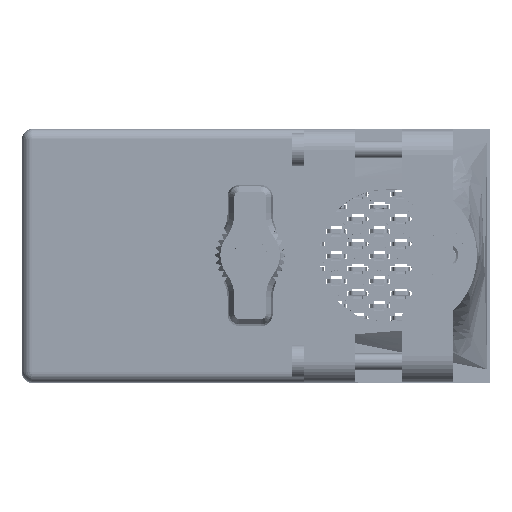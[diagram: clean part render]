
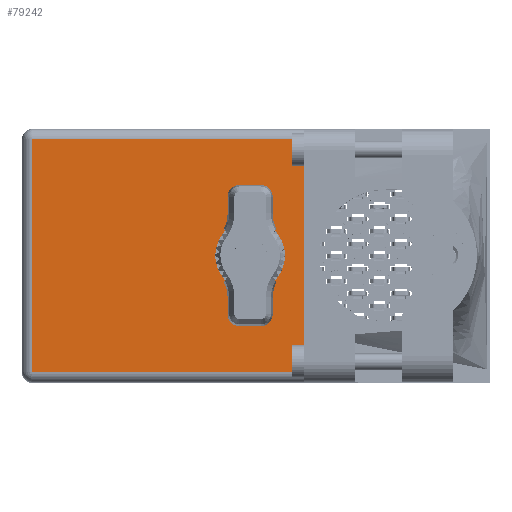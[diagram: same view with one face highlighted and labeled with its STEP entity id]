
A CAD part, top view. The second image highlights one B-rep face of the part: STEP entity #79242.
In plain terms, the highlighted face is planar.
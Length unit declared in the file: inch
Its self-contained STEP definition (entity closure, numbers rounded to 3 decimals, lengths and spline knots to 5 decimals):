
#1709 = DIRECTION ( 'NONE',  ( -1., 0., 0. ) ) ;
#2238 = EDGE_CURVE ( 'NONE', #68252, #86363, #70495, .T. ) ;
#2355 = VERTEX_POINT ( 'NONE', #63988 ) ;
#6141 = EDGE_CURVE ( 'NONE', #2355, #67868, #67649, .T. ) ;
#7275 = CARTESIAN_POINT ( 'NONE',  ( 0.3275, 1.93, 0.703 ) ) ;
#8438 = EDGE_CURVE ( 'NONE', #25638, #2355, #34838, .T. ) ;
#10972 = DIRECTION ( 'NONE',  ( 0., 0., 1. ) ) ;
#18966 = DIRECTION ( 'NONE',  ( 0., 0., 1. ) ) ;
#19156 = AXIS2_PLACEMENT_3D ( 'NONE', #27932, #29498, #1709 ) ;
#25561 = DIRECTION ( 'NONE',  ( 0., 0., 1. ) ) ;
#25638 = VERTEX_POINT ( 'NONE', #112360 ) ;
#27932 = CARTESIAN_POINT ( 'NONE',  ( -1.3775, 1.93, -0.765 ) ) ;
#28512 = EDGE_LOOP ( 'NONE', ( #109829, #52569, #81997, #28928 ) ) ;
#28665 = DIRECTION ( 'NONE',  ( 0., 0., 1. ) ) ;
#28928 = ORIENTED_EDGE ( 'NONE', *, *, #32150, .T. ) ;
#29498 = DIRECTION ( 'NONE',  ( 0., 1., 0. ) ) ;
#29762 = CARTESIAN_POINT ( 'NONE',  ( -1.3155, 1.93, -0.765 ) ) ;
#32150 = EDGE_CURVE ( 'NONE', #102477, #25638, #57107, .T. ) ;
#33489 = AXIS2_PLACEMENT_3D ( 'NONE', #60456, #79254, #25561 ) ;
#34838 = LINE ( 'NONE', #29762, #99309 ) ;
#41670 = CARTESIAN_POINT ( 'NONE',  ( 0.3275, 1.93, -0.703 ) ) ;
#45185 = FACE_OUTER_BOUND ( 'NONE', #28512, .T. ) ;
#47672 = CARTESIAN_POINT ( 'NONE',  ( -1.3775, 1.93, -0.703 ) ) ;
#47710 = CARTESIAN_POINT ( 'NONE',  ( 0.3275, 1.93, 0.703 ) ) ;
#52341 = LINE ( 'NONE', #107904, #83301 ) ;
#52569 = ORIENTED_EDGE ( 'NONE', *, *, #6141, .T. ) ;
#54262 = VECTOR ( 'NONE', #56357, 39.37008 ) ;
#56357 = DIRECTION ( 'NONE',  ( -1., 0., 0. ) ) ;
#57107 = LINE ( 'NONE', #47672, #54262 ) ;
#57628 = EDGE_LOOP ( 'NONE', ( #60915, #113549 ) ) ;
#60456 = CARTESIAN_POINT ( 'NONE',  ( 0., 1.93, 0. ) ) ;
#60651 = FACE_BOUND ( 'NONE', #57628, .T. ) ;
#60915 = ORIENTED_EDGE ( 'NONE', *, *, #2238, .F. ) ;
#62468 = DIRECTION ( 'NONE',  ( 0., 1., 0. ) ) ;
#63988 = CARTESIAN_POINT ( 'NONE',  ( -1.3155, 1.93, 0.703 ) ) ;
#64382 = CARTESIAN_POINT ( 'NONE',  ( 0., 1.93, 0.17 ) ) ;
#64838 = VECTOR ( 'NONE', #69977, 39.37008 ) ;
#67649 = LINE ( 'NONE', #7275, #64838 ) ;
#67868 = VERTEX_POINT ( 'NONE', #47710 ) ;
#68252 = VERTEX_POINT ( 'NONE', #64382 ) ;
#69977 = DIRECTION ( 'NONE',  ( 1., 0., 0. ) ) ;
#70495 = CIRCLE ( 'NONE', #86050, 0.17 ) ;
#78406 = CIRCLE ( 'NONE', #33489, 0.17 ) ;
#79242 = ADVANCED_FACE ( 'NONE', ( #45185, #60651 ), #81624, .T. ) ;
#79254 = DIRECTION ( 'NONE',  ( 0., 1., 0. ) ) ;
#81624 = PLANE ( 'NONE',  #19156 ) ;
#81997 = ORIENTED_EDGE ( 'NONE', *, *, #94929, .F. ) ;
#83301 = VECTOR ( 'NONE', #18966, 39.37008 ) ;
#86050 = AXIS2_PLACEMENT_3D ( 'NONE', #116041, #62468, #28665 ) ;
#86363 = VERTEX_POINT ( 'NONE', #97337 ) ;
#89303 = EDGE_CURVE ( 'NONE', #86363, #68252, #78406, .T. ) ;
#94929 = EDGE_CURVE ( 'NONE', #102477, #67868, #52341, .T. ) ;
#97337 = CARTESIAN_POINT ( 'NONE',  ( 0., 1.93, -0.17 ) ) ;
#99309 = VECTOR ( 'NONE', #10972, 39.37008 ) ;
#102477 = VERTEX_POINT ( 'NONE', #41670 ) ;
#107904 = CARTESIAN_POINT ( 'NONE',  ( 0.3275, 1.93, -0.765 ) ) ;
#109829 = ORIENTED_EDGE ( 'NONE', *, *, #8438, .T. ) ;
#112360 = CARTESIAN_POINT ( 'NONE',  ( -1.3155, 1.93, -0.703 ) ) ;
#113549 = ORIENTED_EDGE ( 'NONE', *, *, #89303, .F. ) ;
#116041 = CARTESIAN_POINT ( 'NONE',  ( 0., 1.93, 0. ) ) ;
